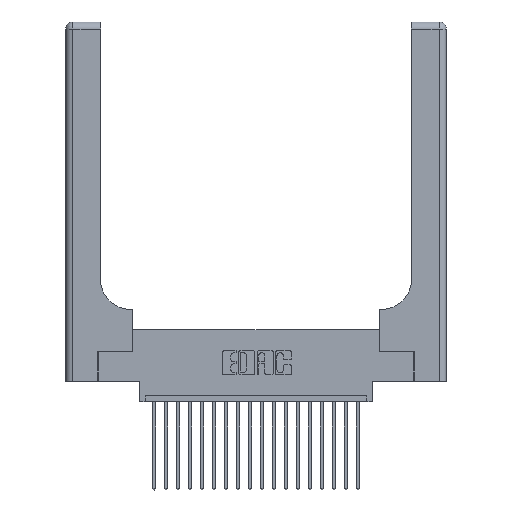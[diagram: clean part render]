
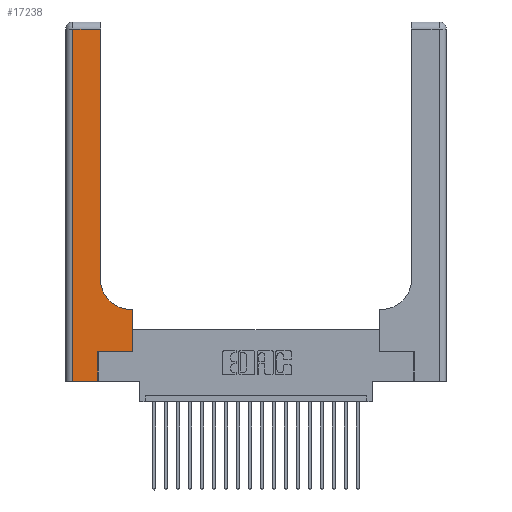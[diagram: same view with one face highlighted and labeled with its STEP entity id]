
A CAD part, top view. The second image highlights one B-rep face of the part: STEP entity #17238.
In plain terms, the highlighted planar face has unit normal (0, 0, 1).
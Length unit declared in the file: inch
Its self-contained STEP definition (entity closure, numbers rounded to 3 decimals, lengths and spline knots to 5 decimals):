
#834 = LINE ( 'NONE', #1785, #13117 ) ;
#1239 = VECTOR ( 'NONE', #18644, 39.37008 ) ;
#1315 = EDGE_CURVE ( 'NONE', #13887, #4421, #834, .T. ) ;
#1521 = LINE ( 'NONE', #15199, #1239 ) ;
#1555 = LINE ( 'NONE', #17624, #8465 ) ;
#1785 = CARTESIAN_POINT ( 'NONE',  ( 0.5585, 0.25, 0.37 ) ) ;
#2152 = EDGE_CURVE ( 'NONE', #19279, #13887, #13866, .T. ) ;
#2832 = CARTESIAN_POINT ( 'NONE',  ( 0.269, 0.25, 0.37 ) ) ;
#2905 = DIRECTION ( 'NONE',  ( -1., 0., 0. ) ) ;
#3239 = CARTESIAN_POINT ( 'NONE',  ( 0.06, 3., 0.37 ) ) ;
#3276 = VERTEX_POINT ( 'NONE', #17666 ) ;
#3312 = DIRECTION ( 'NONE',  ( 0., -1., 0. ) ) ;
#3432 = DIRECTION ( 'NONE',  ( 0., 0., -1. ) ) ;
#4051 = DIRECTION ( 'NONE',  ( -1., 0., 0. ) ) ;
#4154 = EDGE_CURVE ( 'NONE', #13136, #18868, #1555, .T. ) ;
#4341 = EDGE_CURVE ( 'NONE', #4421, #3276, #12735, .T. ) ;
#4343 = AXIS2_PLACEMENT_3D ( 'NONE', #7047, #3432, #15366 ) ;
#4380 = ORIENTED_EDGE ( 'NONE', *, *, #4154, .T. ) ;
#4421 = VERTEX_POINT ( 'NONE', #15701 ) ;
#4758 = LINE ( 'NONE', #9262, #16497 ) ;
#4795 = VECTOR ( 'NONE', #3312, 39.37008 ) ;
#4805 = VECTOR ( 'NONE', #20686, 39.37008 ) ;
#4810 = ORIENTED_EDGE ( 'NONE', *, *, #11610, .T. ) ;
#5607 = EDGE_CURVE ( 'NONE', #3276, #10846, #20162, .T. ) ;
#6339 = DIRECTION ( 'NONE',  ( 0., 0., -1. ) ) ;
#6342 = FACE_OUTER_BOUND ( 'NONE', #9433, .T. ) ;
#6770 = ORIENTED_EDGE ( 'NONE', *, *, #16778, .T. ) ;
#6934 = LINE ( 'NONE', #8397, #10965 ) ;
#6978 = PLANE ( 'NONE',  #4343 ) ;
#7047 = CARTESIAN_POINT ( 'NONE',  ( 0., 3., 0.37 ) ) ;
#7316 = ORIENTED_EDGE ( 'NONE', *, *, #11015, .T. ) ;
#8397 = CARTESIAN_POINT ( 'NONE',  ( 0.2915, 3., 0.37 ) ) ;
#8465 = VECTOR ( 'NONE', #21176, 39.37008 ) ;
#8698 = DIRECTION ( 'NONE',  ( 0., 1., 0. ) ) ;
#9262 = CARTESIAN_POINT ( 'NONE',  ( 0., 2.94, 0.37 ) ) ;
#9433 = EDGE_LOOP ( 'NONE', ( #7316, #6770, #4810, #4380, #14833, #20829, #19864, #9929, #14100 ) ) ;
#9591 = CARTESIAN_POINT ( 'NONE',  ( 0.269, 0.25, 0.37 ) ) ;
#9845 = CARTESIAN_POINT ( 'NONE',  ( 0.2915, 0.6, 0.37 ) ) ;
#9929 = ORIENTED_EDGE ( 'NONE', *, *, #4341, .T. ) ;
#10304 = CARTESIAN_POINT ( 'NONE',  ( 0.5415, 0.85, 0.37 ) ) ;
#10439 = CARTESIAN_POINT ( 'NONE',  ( 0.06, 2.94, 0.37 ) ) ;
#10708 = CARTESIAN_POINT ( 'NONE',  ( 0.5585, 0.25, 0.37 ) ) ;
#10846 = VERTEX_POINT ( 'NONE', #21382 ) ;
#10965 = VECTOR ( 'NONE', #22112, 39.37008 ) ;
#11015 = EDGE_CURVE ( 'NONE', #10846, #14111, #6934, .T. ) ;
#11345 = CARTESIAN_POINT ( 'NONE',  ( 0.06, 0., 0.37 ) ) ;
#11610 = EDGE_CURVE ( 'NONE', #13702, #13136, #18688, .T. ) ;
#12735 = LINE ( 'NONE', #9845, #18352 ) ;
#13117 = VECTOR ( 'NONE', #8698, 39.37008 ) ;
#13136 = VERTEX_POINT ( 'NONE', #11345 ) ;
#13211 = DIRECTION ( 'NONE',  ( 1., 0., 0. ) ) ;
#13289 = CARTESIAN_POINT ( 'NONE',  ( 0.2915, 2.94, 0.37 ) ) ;
#13702 = VERTEX_POINT ( 'NONE', #10439 ) ;
#13866 = LINE ( 'NONE', #9591, #4805 ) ;
#13887 = VERTEX_POINT ( 'NONE', #10708 ) ;
#14100 = ORIENTED_EDGE ( 'NONE', *, *, #5607, .T. ) ;
#14111 = VERTEX_POINT ( 'NONE', #13289 ) ;
#14833 = ORIENTED_EDGE ( 'NONE', *, *, #17804, .T. ) ;
#15199 = CARTESIAN_POINT ( 'NONE',  ( 0.269, 0., 0.37 ) ) ;
#15366 = DIRECTION ( 'NONE',  ( -1., 0., 0. ) ) ;
#15701 = CARTESIAN_POINT ( 'NONE',  ( 0.5585, 0.6, 0.37 ) ) ;
#16497 = VECTOR ( 'NONE', #4051, 39.37008 ) ;
#16778 = EDGE_CURVE ( 'NONE', #14111, #13702, #4758, .T. ) ;
#16889 = CARTESIAN_POINT ( 'NONE',  ( 0.269, 0., 0.37 ) ) ;
#16958 = AXIS2_PLACEMENT_3D ( 'NONE', #10304, #6339, #13211 ) ;
#17238 = ADVANCED_FACE ( 'NONE', ( #6342 ), #6978, .F. ) ;
#17624 = CARTESIAN_POINT ( 'NONE',  ( 0., 0., 0.37 ) ) ;
#17666 = CARTESIAN_POINT ( 'NONE',  ( 0.5415, 0.6, 0.37 ) ) ;
#17804 = EDGE_CURVE ( 'NONE', #18868, #19279, #1521, .T. ) ;
#18352 = VECTOR ( 'NONE', #2905, 39.37008 ) ;
#18644 = DIRECTION ( 'NONE',  ( 0., 1., 0. ) ) ;
#18688 = LINE ( 'NONE', #3239, #4795 ) ;
#18868 = VERTEX_POINT ( 'NONE', #16889 ) ;
#19279 = VERTEX_POINT ( 'NONE', #2832 ) ;
#19864 = ORIENTED_EDGE ( 'NONE', *, *, #1315, .T. ) ;
#20162 = CIRCLE ( 'NONE', #16958, 0.25 ) ;
#20686 = DIRECTION ( 'NONE',  ( 1., 0., 0. ) ) ;
#20829 = ORIENTED_EDGE ( 'NONE', *, *, #2152, .T. ) ;
#21176 = DIRECTION ( 'NONE',  ( 1., 0., 0. ) ) ;
#21382 = CARTESIAN_POINT ( 'NONE',  ( 0.2915, 0.85, 0.37 ) ) ;
#22112 = DIRECTION ( 'NONE',  ( 0., 1., 0. ) ) ;
